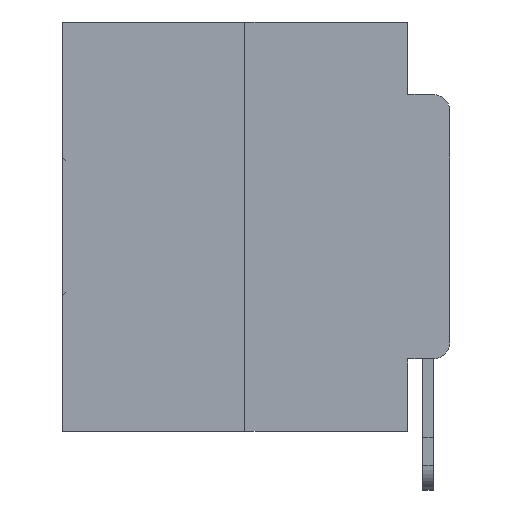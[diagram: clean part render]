
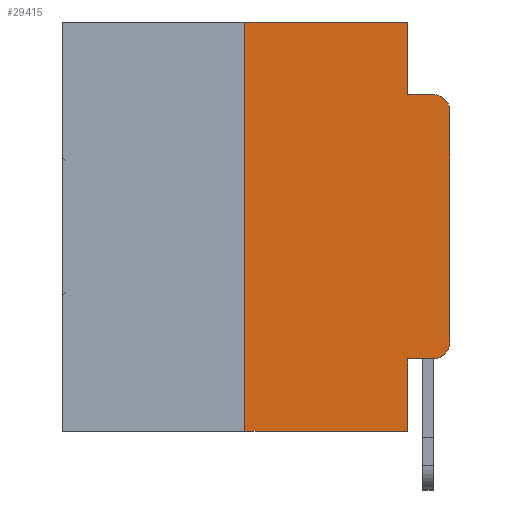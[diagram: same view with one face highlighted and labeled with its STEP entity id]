
A CAD part, left-side view. The second image highlights one B-rep face of the part: STEP entity #29415.
In plain terms, the highlighted planar face has unit normal (-1, 0, 0).
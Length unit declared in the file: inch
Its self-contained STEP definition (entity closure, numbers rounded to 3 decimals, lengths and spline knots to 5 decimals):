
#240 = ORIENTED_EDGE ( 'NONE', *, *, #23858, .T. ) ;
#536 = ORIENTED_EDGE ( 'NONE', *, *, #10971, .F. ) ;
#550 = VERTEX_POINT ( 'NONE', #6492 ) ;
#1898 = VERTEX_POINT ( 'NONE', #13894 ) ;
#2219 = CARTESIAN_POINT ( 'NONE',  ( 0., 0.02, -0.4115 ) ) ;
#3260 = VECTOR ( 'NONE', #17046, 39.37008 ) ;
#3337 = EDGE_CURVE ( 'NONE', #29109, #27534, #9443, .T. ) ;
#3893 = VERTEX_POINT ( 'NONE', #10898 ) ;
#4031 = LINE ( 'NONE', #7398, #3260 ) ;
#4325 = VERTEX_POINT ( 'NONE', #28629 ) ;
#4362 = DIRECTION ( 'NONE',  ( 0., 0., 1. ) ) ;
#4372 = ORIENTED_EDGE ( 'NONE', *, *, #30495, .F. ) ;
#4409 = LINE ( 'NONE', #5108, #10117 ) ;
#4715 = CARTESIAN_POINT ( 'NONE',  ( 0., 0.051, -0.4115 ) ) ;
#5089 = EDGE_CURVE ( 'NONE', #27534, #31513, #15369, .T. ) ;
#5108 = CARTESIAN_POINT ( 'NONE',  ( 0., 0., 0. ) ) ;
#5218 = EDGE_LOOP ( 'NONE', ( #240, #16710, #6566, #536, #4372, #8063, #14337, #8596, #30808, #30796 ) ) ;
#6015 = VECTOR ( 'NONE', #30748, 39.37008 ) ;
#6101 = CARTESIAN_POINT ( 'NONE',  ( 0., 0.473, 0. ) ) ;
#6492 = CARTESIAN_POINT ( 'NONE',  ( 0., 0.051, 0. ) ) ;
#6566 = ORIENTED_EDGE ( 'NONE', *, *, #17063, .F. ) ;
#6945 = CARTESIAN_POINT ( 'NONE',  ( 0., 0., -0.3915 ) ) ;
#7398 = CARTESIAN_POINT ( 'NONE',  ( 0., 0.051, 0. ) ) ;
#8063 = ORIENTED_EDGE ( 'NONE', *, *, #13915, .F. ) ;
#8354 = CARTESIAN_POINT ( 'NONE',  ( 0., 0.02, -0.3915 ) ) ;
#8596 = ORIENTED_EDGE ( 'NONE', *, *, #12904, .F. ) ;
#9058 = VECTOR ( 'NONE', #20889, 39.37008 ) ;
#9164 = DIRECTION ( 'NONE',  ( 0., -1., 0. ) ) ;
#9419 = FACE_OUTER_BOUND ( 'NONE', #5218, .T. ) ;
#9443 = LINE ( 'NONE', #28507, #6015 ) ;
#10117 = VECTOR ( 'NONE', #24320, 39.37008 ) ;
#10898 = CARTESIAN_POINT ( 'NONE',  ( 0., 0.25, -0.5 ) ) ;
#10971 = EDGE_CURVE ( 'NONE', #550, #20261, #16633, .T. ) ;
#11706 = CARTESIAN_POINT ( 'NONE',  ( 0., 0., -0.1085 ) ) ;
#11742 = CARTESIAN_POINT ( 'NONE',  ( 0., 0.02, -0.1085 ) ) ;
#12904 = EDGE_CURVE ( 'NONE', #29109, #1898, #4031, .T. ) ;
#13894 = CARTESIAN_POINT ( 'NONE',  ( 0., 0.051, -0.5 ) ) ;
#13915 = EDGE_CURVE ( 'NONE', #3893, #18210, #15341, .T. ) ;
#14228 = LINE ( 'NONE', #15469, #17987 ) ;
#14290 = EDGE_CURVE ( 'NONE', #3893, #1898, #20256, .T. ) ;
#14337 = ORIENTED_EDGE ( 'NONE', *, *, #14290, .T. ) ;
#15341 = LINE ( 'NONE', #30902, #16492 ) ;
#15369 = CIRCLE ( 'NONE', #24048, 0.02 ) ;
#15469 = CARTESIAN_POINT ( 'NONE',  ( 0., 0.473, 0. ) ) ;
#15636 = PLANE ( 'NONE',  #19180 ) ;
#16097 = VECTOR ( 'NONE', #9164, 39.37008 ) ;
#16267 = CARTESIAN_POINT ( 'NONE',  ( 0., 0.473, -0.5 ) ) ;
#16492 = VECTOR ( 'NONE', #4362, 39.37008 ) ;
#16633 = LINE ( 'NONE', #30843, #9058 ) ;
#16710 = ORIENTED_EDGE ( 'NONE', *, *, #27678, .T. ) ;
#17046 = DIRECTION ( 'NONE',  ( 0., 0., -1. ) ) ;
#17063 = EDGE_CURVE ( 'NONE', #20261, #4325, #31406, .T. ) ;
#17081 = CIRCLE ( 'NONE', #25007, 0.02 ) ;
#17987 = VECTOR ( 'NONE', #20245, 39.37008 ) ;
#18210 = VERTEX_POINT ( 'NONE', #24867 ) ;
#19180 = AXIS2_PLACEMENT_3D ( 'NONE', #6101, #23079, #25172 ) ;
#20245 = DIRECTION ( 'NONE',  ( 0., -1., 0. ) ) ;
#20256 = LINE ( 'NONE', #16267, #16097 ) ;
#20261 = VERTEX_POINT ( 'NONE', #23555 ) ;
#20889 = DIRECTION ( 'NONE',  ( 0., 0., -1. ) ) ;
#21395 = DIRECTION ( 'NONE',  ( -1., 0., 0. ) ) ;
#22675 = DIRECTION ( 'NONE',  ( -1., 0., 0. ) ) ;
#23079 = DIRECTION ( 'NONE',  ( 1., 0., 0. ) ) ;
#23555 = CARTESIAN_POINT ( 'NONE',  ( 0., 0.051, -0.0885 ) ) ;
#23858 = EDGE_CURVE ( 'NONE', #31513, #24263, #4409, .T. ) ;
#24048 = AXIS2_PLACEMENT_3D ( 'NONE', #8354, #22675, #30198 ) ;
#24263 = VERTEX_POINT ( 'NONE', #11706 ) ;
#24320 = DIRECTION ( 'NONE',  ( 0., 0., 1. ) ) ;
#24850 = DIRECTION ( 'NONE',  ( 0., -1., 0. ) ) ;
#24867 = CARTESIAN_POINT ( 'NONE',  ( 0., 0.25, 0. ) ) ;
#25007 = AXIS2_PLACEMENT_3D ( 'NONE', #11742, #21395, #26456 ) ;
#25172 = DIRECTION ( 'NONE',  ( 0., 0., -1. ) ) ;
#26191 = CARTESIAN_POINT ( 'NONE',  ( 0., 0.051, -0.0885 ) ) ;
#26456 = DIRECTION ( 'NONE',  ( 0., 0., -1. ) ) ;
#27217 = VECTOR ( 'NONE', #24850, 39.37008 ) ;
#27534 = VERTEX_POINT ( 'NONE', #2219 ) ;
#27678 = EDGE_CURVE ( 'NONE', #24263, #4325, #17081, .T. ) ;
#28507 = CARTESIAN_POINT ( 'NONE',  ( 0., 0.051, -0.4115 ) ) ;
#28629 = CARTESIAN_POINT ( 'NONE',  ( 0., 0.02, -0.0885 ) ) ;
#29109 = VERTEX_POINT ( 'NONE', #4715 ) ;
#29415 = ADVANCED_FACE ( 'NONE', ( #9419 ), #15636, .F. ) ;
#30198 = DIRECTION ( 'NONE',  ( 0., 0., -1. ) ) ;
#30495 = EDGE_CURVE ( 'NONE', #18210, #550, #14228, .T. ) ;
#30748 = DIRECTION ( 'NONE',  ( 0., -1., 0. ) ) ;
#30796 = ORIENTED_EDGE ( 'NONE', *, *, #5089, .T. ) ;
#30808 = ORIENTED_EDGE ( 'NONE', *, *, #3337, .T. ) ;
#30843 = CARTESIAN_POINT ( 'NONE',  ( 0., 0.051, 0. ) ) ;
#30902 = CARTESIAN_POINT ( 'NONE',  ( 0., 0.25, 0. ) ) ;
#31406 = LINE ( 'NONE', #26191, #27217 ) ;
#31513 = VERTEX_POINT ( 'NONE', #6945 ) ;
